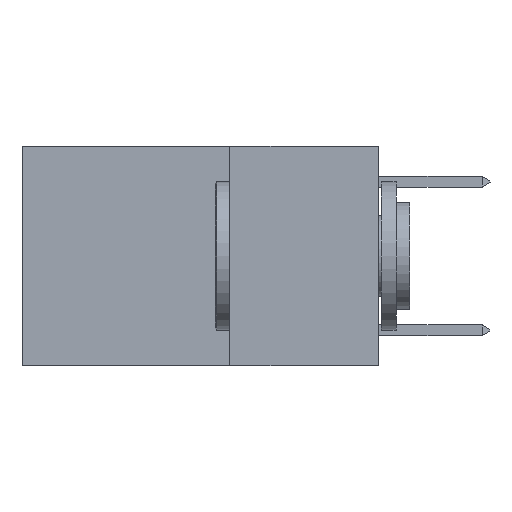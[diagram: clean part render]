
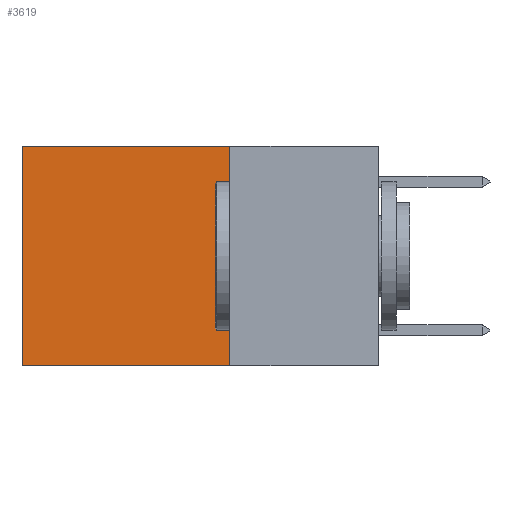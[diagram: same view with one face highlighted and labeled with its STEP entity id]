
A CAD part, left-side view. The second image highlights one B-rep face of the part: STEP entity #3619.
In plain terms, the highlighted planar face has unit normal (-1, 0, 0).
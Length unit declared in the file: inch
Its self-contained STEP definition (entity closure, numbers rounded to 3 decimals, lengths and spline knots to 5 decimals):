
#220 = EDGE_LOOP ( 'NONE', ( #3574, #2957, #5879, #6661 ) ) ;
#449 = DIRECTION ( 'NONE',  ( 0., 1., 0. ) ) ;
#516 = VERTEX_POINT ( 'NONE', #1521 ) ;
#662 = LINE ( 'NONE', #6550, #2809 ) ;
#784 = CARTESIAN_POINT ( 'NONE',  ( 0.2625, 0.25, 0. ) ) ;
#904 = CARTESIAN_POINT ( 'NONE',  ( 0.2625, 0.25, 0. ) ) ;
#1246 = DIRECTION ( 'NONE',  ( 0., 0., -1. ) ) ;
#1521 = CARTESIAN_POINT ( 'NONE',  ( 0.2625, 0.6, 0. ) ) ;
#1778 = VERTEX_POINT ( 'NONE', #8338 ) ;
#2648 = AXIS2_PLACEMENT_3D ( 'NONE', #904, #4334, #5775 ) ;
#2809 = VECTOR ( 'NONE', #449, 39.37008 ) ;
#2957 = ORIENTED_EDGE ( 'NONE', *, *, #5917, .F. ) ;
#3574 = ORIENTED_EDGE ( 'NONE', *, *, #7710, .T. ) ;
#3619 = ADVANCED_FACE ( 'NONE', ( #8048 ), #3674, .F. ) ;
#3674 = PLANE ( 'NONE',  #2648 ) ;
#3980 = CARTESIAN_POINT ( 'NONE',  ( 0.2625, 0.25, 0. ) ) ;
#4003 = CARTESIAN_POINT ( 'NONE',  ( 0.2625, 0.6, 0. ) ) ;
#4109 = LINE ( 'NONE', #4003, #9029 ) ;
#4183 = CARTESIAN_POINT ( 'NONE',  ( 0.2625, 0.25, -0.37 ) ) ;
#4334 = DIRECTION ( 'NONE',  ( 1., 0., 0. ) ) ;
#4356 = LINE ( 'NONE', #784, #6331 ) ;
#4416 = LINE ( 'NONE', #6546, #6390 ) ;
#5775 = DIRECTION ( 'NONE',  ( 0., 0., -1. ) ) ;
#5879 = ORIENTED_EDGE ( 'NONE', *, *, #7285, .F. ) ;
#5917 = EDGE_CURVE ( 'NONE', #7360, #1778, #662, .T. ) ;
#6331 = VECTOR ( 'NONE', #6963, 39.37008 ) ;
#6390 = VECTOR ( 'NONE', #6572, 39.37008 ) ;
#6546 = CARTESIAN_POINT ( 'NONE',  ( 0.2625, 0.25, 0. ) ) ;
#6550 = CARTESIAN_POINT ( 'NONE',  ( 0.2625, 0.25, -0.37 ) ) ;
#6572 = DIRECTION ( 'NONE',  ( 0., 1., 0. ) ) ;
#6661 = ORIENTED_EDGE ( 'NONE', *, *, #8753, .T. ) ;
#6963 = DIRECTION ( 'NONE',  ( 0., 0., -1. ) ) ;
#7151 = VERTEX_POINT ( 'NONE', #3980 ) ;
#7285 = EDGE_CURVE ( 'NONE', #7151, #7360, #4356, .T. ) ;
#7360 = VERTEX_POINT ( 'NONE', #4183 ) ;
#7710 = EDGE_CURVE ( 'NONE', #516, #1778, #4109, .T. ) ;
#8048 = FACE_OUTER_BOUND ( 'NONE', #220, .T. ) ;
#8338 = CARTESIAN_POINT ( 'NONE',  ( 0.2625, 0.6, -0.37 ) ) ;
#8753 = EDGE_CURVE ( 'NONE', #7151, #516, #4416, .T. ) ;
#9029 = VECTOR ( 'NONE', #1246, 39.37008 ) ;
